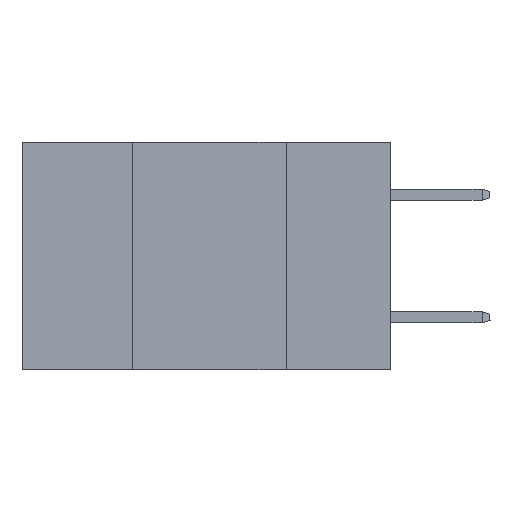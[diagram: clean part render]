
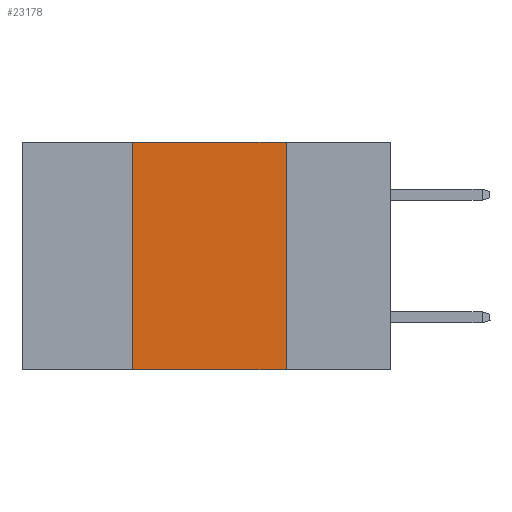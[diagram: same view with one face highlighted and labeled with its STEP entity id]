
A CAD part, left-side view. The second image highlights one B-rep face of the part: STEP entity #23178.
In plain terms, the highlighted planar face has unit normal (-1, 0, 0).
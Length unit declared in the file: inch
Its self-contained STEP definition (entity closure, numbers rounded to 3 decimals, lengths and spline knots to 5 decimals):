
#1601 = CARTESIAN_POINT ( 'NONE',  ( 0., 0.6, 0. ) ) ;
#3701 = AXIS2_PLACEMENT_3D ( 'NONE', #1601, #12532, #10181 ) ;
#3998 = EDGE_CURVE ( 'NONE', #5586, #27557, #6660, .T. ) ;
#4061 = VECTOR ( 'NONE', #26378, 39.37008 ) ;
#4426 = CARTESIAN_POINT ( 'NONE',  ( 0., 0.6, -0.37 ) ) ;
#5586 = VERTEX_POINT ( 'NONE', #18345 ) ;
#5880 = CARTESIAN_POINT ( 'NONE',  ( 0., 0.42, 0. ) ) ;
#6660 = LINE ( 'NONE', #23483, #9026 ) ;
#7834 = FACE_OUTER_BOUND ( 'NONE', #13556, .T. ) ;
#8198 = ORIENTED_EDGE ( 'NONE', *, *, #20799, .F. ) ;
#8525 = DIRECTION ( 'NONE',  ( 0., -1., 0. ) ) ;
#8672 = CARTESIAN_POINT ( 'NONE',  ( 0., 0.17, 0. ) ) ;
#9026 = VECTOR ( 'NONE', #8525, 39.37008 ) ;
#10181 = DIRECTION ( 'NONE',  ( 0., 0., -1. ) ) ;
#10379 = PLANE ( 'NONE',  #3701 ) ;
#11090 = VERTEX_POINT ( 'NONE', #26601 ) ;
#11147 = LINE ( 'NONE', #4426, #4061 ) ;
#12367 = ORIENTED_EDGE ( 'NONE', *, *, #22662, .F. ) ;
#12532 = DIRECTION ( 'NONE',  ( 1., 0., 0. ) ) ;
#13411 = VECTOR ( 'NONE', #21247, 39.37008 ) ;
#13556 = EDGE_LOOP ( 'NONE', ( #8198, #19413, #12367, #22276 ) ) ;
#14641 = VECTOR ( 'NONE', #23188, 39.37008 ) ;
#18345 = CARTESIAN_POINT ( 'NONE',  ( 0., 0.42, 0. ) ) ;
#18526 = EDGE_CURVE ( 'NONE', #11090, #25556, #11147, .T. ) ;
#19037 = CARTESIAN_POINT ( 'NONE',  ( 0., 0.17, -0.37 ) ) ;
#19413 = ORIENTED_EDGE ( 'NONE', *, *, #3998, .F. ) ;
#20762 = LINE ( 'NONE', #5880, #14641 ) ;
#20799 = EDGE_CURVE ( 'NONE', #27557, #25556, #21558, .T. ) ;
#21247 = DIRECTION ( 'NONE',  ( 0., 0., -1. ) ) ;
#21558 = LINE ( 'NONE', #27402, #13411 ) ;
#22276 = ORIENTED_EDGE ( 'NONE', *, *, #18526, .T. ) ;
#22662 = EDGE_CURVE ( 'NONE', #11090, #5586, #20762, .T. ) ;
#23178 = ADVANCED_FACE ( 'NONE', ( #7834 ), #10379, .F. ) ;
#23188 = DIRECTION ( 'NONE',  ( 0., 0., 1. ) ) ;
#23483 = CARTESIAN_POINT ( 'NONE',  ( 0., 0.6, 0. ) ) ;
#25556 = VERTEX_POINT ( 'NONE', #19037 ) ;
#26378 = DIRECTION ( 'NONE',  ( 0., -1., 0. ) ) ;
#26601 = CARTESIAN_POINT ( 'NONE',  ( 0., 0.42, -0.37 ) ) ;
#27402 = CARTESIAN_POINT ( 'NONE',  ( 0., 0.17, 0. ) ) ;
#27557 = VERTEX_POINT ( 'NONE', #8672 ) ;
